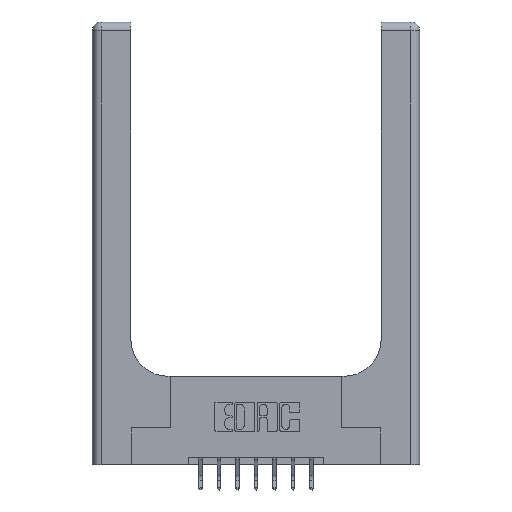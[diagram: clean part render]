
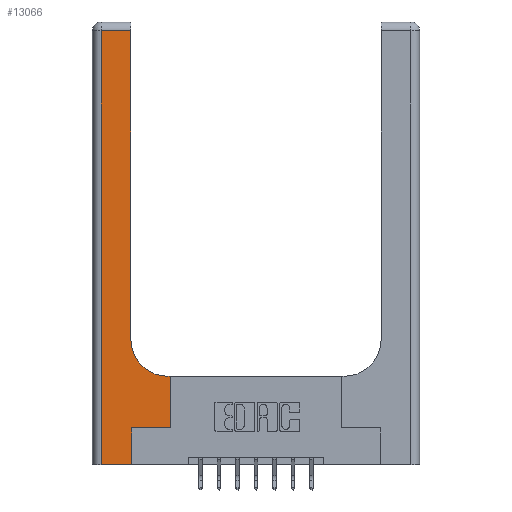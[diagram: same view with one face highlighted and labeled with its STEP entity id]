
A CAD part, top view. The second image highlights one B-rep face of the part: STEP entity #13066.
In plain terms, the highlighted planar face has unit normal (0, 0, 1).
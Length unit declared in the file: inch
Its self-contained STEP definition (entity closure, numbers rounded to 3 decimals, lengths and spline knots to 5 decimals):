
#244 = VERTEX_POINT ( 'NONE', #5886 ) ;
#261 = DIRECTION ( 'NONE',  ( -1., 0., 0. ) ) ;
#269 = CARTESIAN_POINT ( 'NONE',  ( 0.265, 0., 0.37 ) ) ;
#393 = LINE ( 'NONE', #8470, #4609 ) ;
#599 = ORIENTED_EDGE ( 'NONE', *, *, #5013, .T. ) ;
#723 = ORIENTED_EDGE ( 'NONE', *, *, #13994, .T. ) ;
#743 = LINE ( 'NONE', #10251, #2084 ) ;
#1370 = VERTEX_POINT ( 'NONE', #11599 ) ;
#1773 = DIRECTION ( 'NONE',  ( 1., 0., 0. ) ) ;
#1933 = VECTOR ( 'NONE', #4544, 39.37008 ) ;
#2084 = VECTOR ( 'NONE', #14974, 39.37008 ) ;
#2238 = EDGE_CURVE ( 'NONE', #4567, #3097, #14993, .T. ) ;
#2374 = CARTESIAN_POINT ( 'NONE',  ( 0.528, 0.6, 0.37 ) ) ;
#2508 = CARTESIAN_POINT ( 'NONE',  ( 0.51, 0.6, 0.37 ) ) ;
#2670 = LINE ( 'NONE', #269, #11667 ) ;
#2834 = ORIENTED_EDGE ( 'NONE', *, *, #12519, .T. ) ;
#3021 = ORIENTED_EDGE ( 'NONE', *, *, #6527, .T. ) ;
#3097 = VERTEX_POINT ( 'NONE', #4476 ) ;
#3417 = EDGE_CURVE ( 'NONE', #3097, #244, #13458, .T. ) ;
#4290 = EDGE_CURVE ( 'NONE', #6312, #6311, #8490, .T. ) ;
#4357 = DIRECTION ( 'NONE',  ( 0., 1., 0. ) ) ;
#4439 = CARTESIAN_POINT ( 'NONE',  ( 0.26, 3., 0.37 ) ) ;
#4476 = CARTESIAN_POINT ( 'NONE',  ( 0.06, 0., 0.37 ) ) ;
#4478 = VECTOR ( 'NONE', #261, 39.37008 ) ;
#4544 = DIRECTION ( 'NONE',  ( 1., 0., 0. ) ) ;
#4567 = VERTEX_POINT ( 'NONE', #10523 ) ;
#4601 = VECTOR ( 'NONE', #5605, 39.37008 ) ;
#4609 = VECTOR ( 'NONE', #6158, 39.37008 ) ;
#4736 = CIRCLE ( 'NONE', #13262, 0.25 ) ;
#4943 = DIRECTION ( 'NONE',  ( 0., 1., 0. ) ) ;
#4993 = CARTESIAN_POINT ( 'NONE',  ( 0.51, 0.85, 0.37 ) ) ;
#5013 = EDGE_CURVE ( 'NONE', #6278, #1370, #7522, .T. ) ;
#5028 = CARTESIAN_POINT ( 'NONE',  ( 0.528, 0.25, 0.37 ) ) ;
#5086 = VECTOR ( 'NONE', #7351, 39.37008 ) ;
#5131 = EDGE_CURVE ( 'NONE', #6311, #9156, #393, .T. ) ;
#5315 = VECTOR ( 'NONE', #4357, 39.37008 ) ;
#5605 = DIRECTION ( 'NONE',  ( 0., -1., 0. ) ) ;
#5863 = ORIENTED_EDGE ( 'NONE', *, *, #10897, .T. ) ;
#5886 = CARTESIAN_POINT ( 'NONE',  ( 0.265, 0., 0.37 ) ) ;
#6015 = CARTESIAN_POINT ( 'NONE',  ( 0., 3., 0.37 ) ) ;
#6158 = DIRECTION ( 'NONE',  ( -1., 0., 0. ) ) ;
#6278 = VERTEX_POINT ( 'NONE', #13890 ) ;
#6311 = VERTEX_POINT ( 'NONE', #2374 ) ;
#6312 = VERTEX_POINT ( 'NONE', #7963 ) ;
#6527 = EDGE_CURVE ( 'NONE', #244, #10656, #2670, .T. ) ;
#6635 = ORIENTED_EDGE ( 'NONE', *, *, #3417, .T. ) ;
#6937 = DIRECTION ( 'NONE',  ( -1., 0., 0. ) ) ;
#7351 = DIRECTION ( 'NONE',  ( 0., 1., 0. ) ) ;
#7522 = LINE ( 'NONE', #4439, #5315 ) ;
#7963 = CARTESIAN_POINT ( 'NONE',  ( 0.528, 0.25, 0.37 ) ) ;
#8262 = CARTESIAN_POINT ( 'NONE',  ( 0., 2.94, 0.37 ) ) ;
#8470 = CARTESIAN_POINT ( 'NONE',  ( 0.26, 0.6, 0.37 ) ) ;
#8490 = LINE ( 'NONE', #5028, #5086 ) ;
#9156 = VERTEX_POINT ( 'NONE', #2508 ) ;
#9206 = ORIENTED_EDGE ( 'NONE', *, *, #5131, .T. ) ;
#10251 = CARTESIAN_POINT ( 'NONE',  ( 0.265, 0.25, 0.37 ) ) ;
#10523 = CARTESIAN_POINT ( 'NONE',  ( 0.06, 2.94, 0.37 ) ) ;
#10589 = DIRECTION ( 'NONE',  ( 0., 0., -1. ) ) ;
#10656 = VERTEX_POINT ( 'NONE', #11653 ) ;
#10747 = LINE ( 'NONE', #8262, #4478 ) ;
#10788 = ORIENTED_EDGE ( 'NONE', *, *, #2238, .T. ) ;
#10897 = EDGE_CURVE ( 'NONE', #9156, #6278, #4736, .T. ) ;
#11012 = DIRECTION ( 'NONE',  ( 0., 0., -1. ) ) ;
#11599 = CARTESIAN_POINT ( 'NONE',  ( 0.26, 2.94, 0.37 ) ) ;
#11653 = CARTESIAN_POINT ( 'NONE',  ( 0.265, 0.25, 0.37 ) ) ;
#11667 = VECTOR ( 'NONE', #4943, 39.37008 ) ;
#11814 = PLANE ( 'NONE',  #13466 ) ;
#12519 = EDGE_CURVE ( 'NONE', #10656, #6312, #743, .T. ) ;
#12556 = CARTESIAN_POINT ( 'NONE',  ( 0., 0., 0.37 ) ) ;
#12694 = EDGE_LOOP ( 'NONE', ( #599, #723, #10788, #6635, #3021, #2834, #14961, #9206, #5863 ) ) ;
#13066 = ADVANCED_FACE ( 'NONE', ( #13939 ), #11814, .F. ) ;
#13262 = AXIS2_PLACEMENT_3D ( 'NONE', #4993, #11012, #1773 ) ;
#13458 = LINE ( 'NONE', #12556, #1933 ) ;
#13466 = AXIS2_PLACEMENT_3D ( 'NONE', #6015, #10589, #6937 ) ;
#13761 = CARTESIAN_POINT ( 'NONE',  ( 0.06, 3., 0.37 ) ) ;
#13890 = CARTESIAN_POINT ( 'NONE',  ( 0.26, 0.85, 0.37 ) ) ;
#13939 = FACE_OUTER_BOUND ( 'NONE', #12694, .T. ) ;
#13994 = EDGE_CURVE ( 'NONE', #1370, #4567, #10747, .T. ) ;
#14961 = ORIENTED_EDGE ( 'NONE', *, *, #4290, .T. ) ;
#14974 = DIRECTION ( 'NONE',  ( 1., 0., 0. ) ) ;
#14993 = LINE ( 'NONE', #13761, #4601 ) ;
